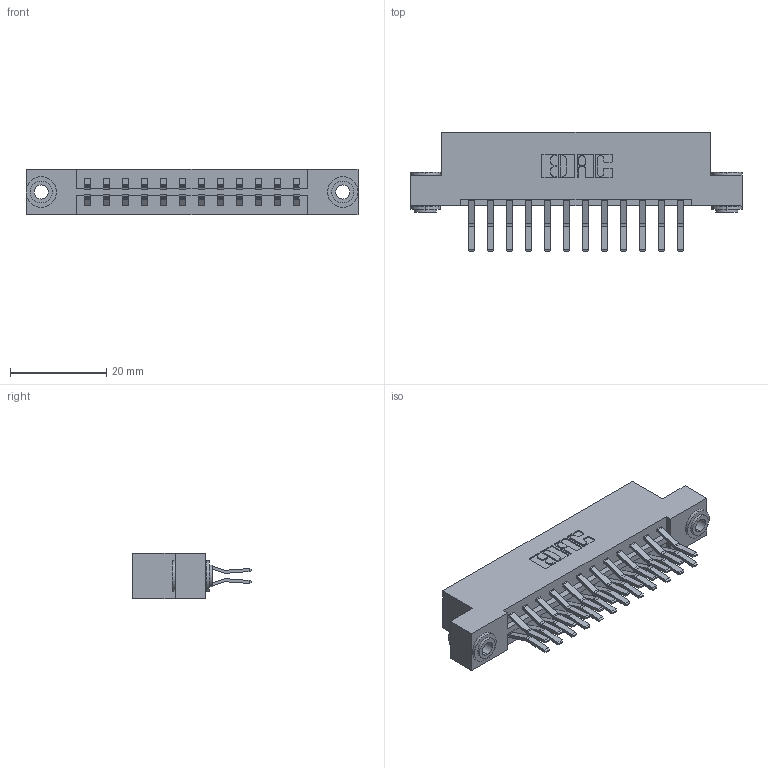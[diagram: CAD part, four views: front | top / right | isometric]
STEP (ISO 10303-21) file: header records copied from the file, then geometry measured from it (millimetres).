
FILE_DESCRIPTION (( 'STEP AP203' ), '1' );
FILE_NAME ('333-024-560-203.STEP', '2018-08-02T11:49:50', ( '' ), ( '' ), 'SwSTEP 2.0', 'SolidWorks 2016', '' );
FILE_SCHEMA (( 'CONFIG_CONTROL_DESIGN' ));
Length unit declared in the file: inch
Products named in the file (4): 345-292-001_560 Tail; 345-250-002_345-250-002-102; 333-024-560-203; 333 Part_Flush - .156 Dia - TH
Assembly tree (27 placements, depth 2):
  333-024-560-203
    333 Part_Flush - .156 Dia - TH
    345-292-001_560 Tail  x24
    345-250-002_345-250-002-102  x2
Bounding box: 69.09 x 24.78 x 9.4 mm (x, y, z)
Volume: 6949.6 mm3; surface area: 8563.5 mm2
Topology: 27 solids, 27 shells, 1448 faces, 4251 edges, 2798 vertices
Faces by surface type: plane 944, cylinder 496, cone 8
Entity records: 12338 total; most frequent: CARTESIAN_POINT 2057, ORIENTED_EDGE 1986, DIRECTION 1847, EDGE_CURVE 993, LINE 837, VECTOR 837, VERTEX_POINT 658, AXIS2_PLACEMENT_3D 505
